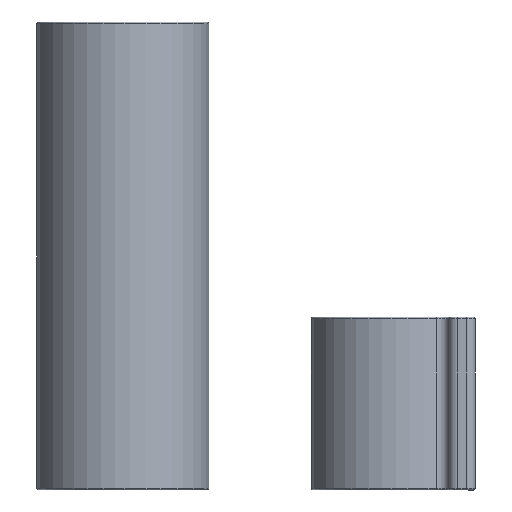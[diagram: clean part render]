
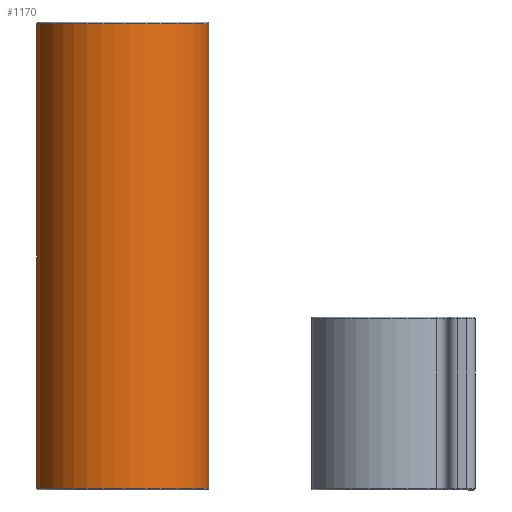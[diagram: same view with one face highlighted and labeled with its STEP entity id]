
A CAD part, left-side view. The second image highlights one B-rep face of the part: STEP entity #1170.
In plain terms, the highlighted cylindrical face has radius 10 mm (diameter 20 mm), a partial arc.
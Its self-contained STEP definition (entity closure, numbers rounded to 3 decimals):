
#91=FACE_OUTER_BOUND('',#170,.T.);
#170=EDGE_LOOP('',(#792,#793,#794,#795));
#253=LINE('',#1966,#311);
#254=LINE('',#1969,#312);
#311=VECTOR('',#1518,10.);
#312=VECTOR('',#1521,10.);
#378=CIRCLE('',#1289,10.);
#379=CIRCLE('',#1291,10.);
#485=VERTEX_POINT('',#1941);
#492=VERTEX_POINT('',#1957);
#493=VERTEX_POINT('',#1965);
#494=VERTEX_POINT('',#1967);
#604=EDGE_CURVE('',#485,#492,#378,.T.);
#605=EDGE_CURVE('',#493,#485,#253,.T.);
#606=EDGE_CURVE('',#494,#493,#379,.T.);
#607=EDGE_CURVE('',#492,#494,#254,.T.);
#792=ORIENTED_EDGE('',*,*,#604,.F.);
#793=ORIENTED_EDGE('',*,*,#605,.F.);
#794=ORIENTED_EDGE('',*,*,#606,.F.);
#795=ORIENTED_EDGE('',*,*,#607,.F.);
#1133=CYLINDRICAL_SURFACE('',#1290,10.);
#1170=ADVANCED_FACE('',(#91),#1133,.T.);
#1289=AXIS2_PLACEMENT_3D('',#1963,#1514,#1515);
#1290=AXIS2_PLACEMENT_3D('',#1964,#1516,#1517);
#1291=AXIS2_PLACEMENT_3D('',#1968,#1519,#1520);
#1514=DIRECTION('center_axis',(0.,0.,
1.));
#1515=DIRECTION('ref_axis',(-1.,0.,0.));
#1516=DIRECTION('center_axis',(0.,0.,
-1.));
#1517=DIRECTION('ref_axis',(0.,-1.,0.));
#1518=DIRECTION('',(0.,0.,1.));
#1519=DIRECTION('center_axis',(0.,0.,
-1.));
#1520=DIRECTION('ref_axis',(-1.,0.,0.));
#1521=DIRECTION('',(0.,0.,-1.));
#1941=CARTESIAN_POINT('',(-1.111,9.938,53.95));
#1957=CARTESIAN_POINT('',(-1.111,-9.938,53.95));
#1963=CARTESIAN_POINT('Origin',(0.,0.,
53.95));
#1964=CARTESIAN_POINT('Origin',(0.,0.,
52.075));
#1965=CARTESIAN_POINT('',(-1.111,9.938,0.2));
#1966=CARTESIAN_POINT('',(-1.111,9.938,52.075));
#1967=CARTESIAN_POINT('',(-1.111,-9.938,0.2));
#1968=CARTESIAN_POINT('Origin',(0.,0.,
0.2));
#1969=CARTESIAN_POINT('',(-1.111,-9.938,52.075));
